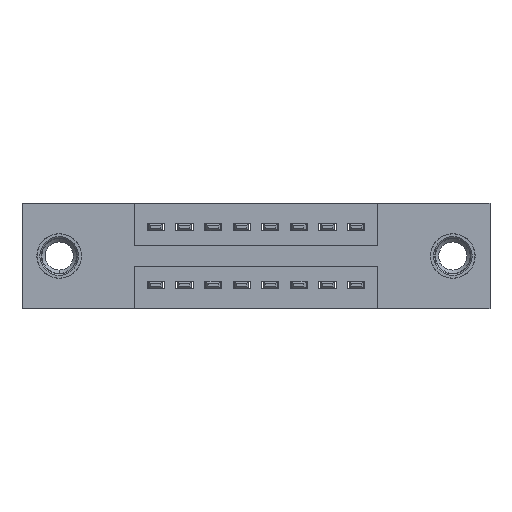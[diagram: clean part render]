
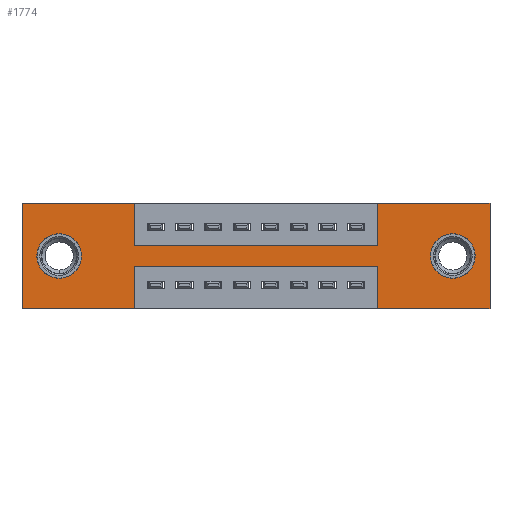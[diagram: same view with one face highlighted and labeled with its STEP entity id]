
A CAD part, front view. The second image highlights one B-rep face of the part: STEP entity #1774.
In plain terms, the highlighted planar face has unit normal (0, -1, 0).
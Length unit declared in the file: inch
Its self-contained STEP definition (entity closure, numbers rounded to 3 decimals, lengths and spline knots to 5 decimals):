
#6 = ORIENTED_EDGE ( 'NONE', *, *, #5524, .T. ) ;
#13 = VERTEX_POINT ( 'NONE', #3725 ) ;
#66 = EDGE_CURVE ( 'NONE', #8561, #3732, #9555, .T. ) ;
#76 = ORIENTED_EDGE ( 'NONE', *, *, #7674, .F. ) ;
#367 = ORIENTED_EDGE ( 'NONE', *, *, #10205, .F. ) ;
#395 = VERTEX_POINT ( 'NONE', #7832 ) ;
#459 = ORIENTED_EDGE ( 'NONE', *, *, #5177, .F. ) ;
#514 = LINE ( 'NONE', #8436, #5668 ) ;
#720 = DIRECTION ( 'NONE',  ( 1., 0., 0. ) ) ;
#758 = EDGE_CURVE ( 'NONE', #3732, #9157, #6215, .T. ) ;
#773 = FACE_BOUND ( 'NONE', #6918, .T. ) ;
#788 = ORIENTED_EDGE ( 'NONE', *, *, #1608, .T. ) ;
#1015 = VERTEX_POINT ( 'NONE', #11795 ) ;
#1145 = VECTOR ( 'NONE', #6794, 39.37008 ) ;
#1333 = CARTESIAN_POINT ( 'NONE',  ( 0., 0., 0. ) ) ;
#1350 = DIRECTION ( 'NONE',  ( 0., 1., 0. ) ) ;
#1471 = ORIENTED_EDGE ( 'NONE', *, *, #9600, .F. ) ;
#1476 = EDGE_CURVE ( 'NONE', #9157, #395, #10089, .T. ) ;
#1489 = DIRECTION ( 'NONE',  ( 0., 0., -1. ) ) ;
#1569 = VERTEX_POINT ( 'NONE', #2866 ) ;
#1586 = CARTESIAN_POINT ( 'NONE',  ( 1.2425, 0., 0. ) ) ;
#1608 = EDGE_CURVE ( 'NONE', #1569, #13, #11328, .T. ) ;
#1685 = CARTESIAN_POINT ( 'NONE',  ( 1.505, 0., -0.185 ) ) ;
#1750 = CIRCLE ( 'NONE', #9805, 0.078 ) ;
#1774 = ADVANCED_FACE ( 'NONE', ( #7945, #773, #5615 ), #3013, .T. ) ;
#1789 = CARTESIAN_POINT ( 'NONE',  ( 0., 0., 0. ) ) ;
#1961 = ORIENTED_EDGE ( 'NONE', *, *, #1476, .F. ) ;
#2021 = ORIENTED_EDGE ( 'NONE', *, *, #2684, .T. ) ;
#2031 = LINE ( 'NONE', #1333, #7217 ) ;
#2106 = ORIENTED_EDGE ( 'NONE', *, *, #9376, .F. ) ;
#2152 = EDGE_CURVE ( 'NONE', #13, #1569, #4315, .T. ) ;
#2191 = ORIENTED_EDGE ( 'NONE', *, *, #2152, .T. ) ;
#2216 = VERTEX_POINT ( 'NONE', #6932 ) ;
#2254 = CARTESIAN_POINT ( 'NONE',  ( 1.2425, 0., -0.22 ) ) ;
#2636 = ORIENTED_EDGE ( 'NONE', *, *, #10783, .F. ) ;
#2684 = EDGE_CURVE ( 'NONE', #5023, #7451, #8291, .T. ) ;
#2705 = LINE ( 'NONE', #7246, #4887 ) ;
#2793 = CARTESIAN_POINT ( 'NONE',  ( 1.2425, 0., -0.15 ) ) ;
#2866 = CARTESIAN_POINT ( 'NONE',  ( 1.505, 0., -0.263 ) ) ;
#2899 = DIRECTION ( 'NONE',  ( 0., 0., -1. ) ) ;
#2922 = VECTOR ( 'NONE', #720, 39.37008 ) ;
#2944 = AXIS2_PLACEMENT_3D ( 'NONE', #1685, #1350, #1489 ) ;
#3013 = PLANE ( 'NONE',  #8326 ) ;
#3107 = DIRECTION ( 'NONE',  ( 0., 0., -1. ) ) ;
#3128 = CARTESIAN_POINT ( 'NONE',  ( 0.13, 0., -0.185 ) ) ;
#3194 = DIRECTION ( 'NONE',  ( 0., 0., -1. ) ) ;
#3308 = DIRECTION ( 'NONE',  ( 0., -1., 0. ) ) ;
#3347 = CARTESIAN_POINT ( 'NONE',  ( 0., 0., -0.37 ) ) ;
#3351 = VERTEX_POINT ( 'NONE', #1586 ) ;
#3572 = VERTEX_POINT ( 'NONE', #11806 ) ;
#3608 = VECTOR ( 'NONE', #2899, 39.37008 ) ;
#3664 = CARTESIAN_POINT ( 'NONE',  ( 0.3925, 0., -0.37 ) ) ;
#3669 = VECTOR ( 'NONE', #4678, 39.37008 ) ;
#3725 = CARTESIAN_POINT ( 'NONE',  ( 1.505, 0., -0.107 ) ) ;
#3732 = VERTEX_POINT ( 'NONE', #2254 ) ;
#3815 = ORIENTED_EDGE ( 'NONE', *, *, #4090, .F. ) ;
#4055 = DIRECTION ( 'NONE',  ( 0., 0., 1. ) ) ;
#4090 = EDGE_CURVE ( 'NONE', #395, #11624, #11880, .T. ) ;
#4171 = ORIENTED_EDGE ( 'NONE', *, *, #66, .F. ) ;
#4315 = CIRCLE ( 'NONE', #8680, 0.078 ) ;
#4380 = CARTESIAN_POINT ( 'NONE',  ( 1.2425, 0., 0. ) ) ;
#4478 = CARTESIAN_POINT ( 'NONE',  ( 0., 0., -0.37 ) ) ;
#4615 = ORIENTED_EDGE ( 'NONE', *, *, #758, .F. ) ;
#4678 = DIRECTION ( 'NONE',  ( 0., 0., 1. ) ) ;
#4767 = EDGE_LOOP ( 'NONE', ( #2191, #788 ) ) ;
#4857 = CARTESIAN_POINT ( 'NONE',  ( 1.2425, 0., -0.37 ) ) ;
#4887 = VECTOR ( 'NONE', #11569, 39.37008 ) ;
#4925 = VECTOR ( 'NONE', #5820, 39.37008 ) ;
#5023 = VERTEX_POINT ( 'NONE', #11286 ) ;
#5134 = CARTESIAN_POINT ( 'NONE',  ( 0.3925, 0., -0.22 ) ) ;
#5177 = EDGE_CURVE ( 'NONE', #3351, #2216, #7677, .T. ) ;
#5264 = VERTEX_POINT ( 'NONE', #2793 ) ;
#5354 = AXIS2_PLACEMENT_3D ( 'NONE', #8125, #8090, #8054 ) ;
#5524 = EDGE_CURVE ( 'NONE', #7451, #5023, #1750, .T. ) ;
#5549 = CARTESIAN_POINT ( 'NONE',  ( 0.3925, 0., -0.15 ) ) ;
#5615 = FACE_OUTER_BOUND ( 'NONE', #7780, .T. ) ;
#5657 = LINE ( 'NONE', #5549, #2922 ) ;
#5668 = VECTOR ( 'NONE', #3107, 39.37008 ) ;
#5820 = DIRECTION ( 'NONE',  ( 0., 0., 1. ) ) ;
#5823 = LINE ( 'NONE', #1789, #3669 ) ;
#5928 = EDGE_CURVE ( 'NONE', #10672, #8561, #2705, .T. ) ;
#6215 = LINE ( 'NONE', #10726, #1145 ) ;
#6374 = CARTESIAN_POINT ( 'NONE',  ( 1.635, 0., 0. ) ) ;
#6794 = DIRECTION ( 'NONE',  ( -1., 0., 0. ) ) ;
#6808 = LINE ( 'NONE', #4380, #7065 ) ;
#6905 = EDGE_CURVE ( 'NONE', #1015, #10204, #2031, .T. ) ;
#6918 = EDGE_LOOP ( 'NONE', ( #2021, #6 ) ) ;
#6932 = CARTESIAN_POINT ( 'NONE',  ( 1.635, 0., 0. ) ) ;
#6963 = CARTESIAN_POINT ( 'NONE',  ( 1.635, 0., -0.37 ) ) ;
#7065 = VECTOR ( 'NONE', #8739, 39.37008 ) ;
#7217 = VECTOR ( 'NONE', #7816, 39.37008 ) ;
#7246 = CARTESIAN_POINT ( 'NONE',  ( 0., 0., -0.37 ) ) ;
#7286 = VECTOR ( 'NONE', #9884, 39.37008 ) ;
#7451 = VERTEX_POINT ( 'NONE', #8423 ) ;
#7674 = EDGE_CURVE ( 'NONE', #2216, #10672, #8265, .T. ) ;
#7677 = LINE ( 'NONE', #8065, #11735 ) ;
#7780 = EDGE_LOOP ( 'NONE', ( #1961, #4615, #4171, #10823, #76, #459, #2636, #367, #1471, #8094, #2106, #3815 ) ) ;
#7816 = DIRECTION ( 'NONE',  ( 1., 0., 0. ) ) ;
#7832 = CARTESIAN_POINT ( 'NONE',  ( 0.3925, 0., -0.37 ) ) ;
#7945 = FACE_BOUND ( 'NONE', #4767, .T. ) ;
#8054 = DIRECTION ( 'NONE',  ( 0., 0., 1. ) ) ;
#8065 = CARTESIAN_POINT ( 'NONE',  ( 0., 0., 0. ) ) ;
#8090 = DIRECTION ( 'NONE',  ( 0., 1., 0. ) ) ;
#8094 = ORIENTED_EDGE ( 'NONE', *, *, #6905, .F. ) ;
#8125 = CARTESIAN_POINT ( 'NONE',  ( 0.13, 0., -0.185 ) ) ;
#8265 = LINE ( 'NONE', #6374, #10593 ) ;
#8291 = CIRCLE ( 'NONE', #5354, 0.078 ) ;
#8326 = AXIS2_PLACEMENT_3D ( 'NONE', #3347, #3308, #3194 ) ;
#8423 = CARTESIAN_POINT ( 'NONE',  ( 0.13, 0., -0.263 ) ) ;
#8436 = CARTESIAN_POINT ( 'NONE',  ( 0.3925, 0., 0. ) ) ;
#8561 = VERTEX_POINT ( 'NONE', #10278 ) ;
#8680 = AXIS2_PLACEMENT_3D ( 'NONE', #9238, #9250, #9213 ) ;
#8739 = DIRECTION ( 'NONE',  ( 0., 0., 1. ) ) ;
#8992 = CARTESIAN_POINT ( 'NONE',  ( 0., 0., -0.37 ) ) ;
#9157 = VERTEX_POINT ( 'NONE', #5134 ) ;
#9213 = DIRECTION ( 'NONE',  ( 0., 0., -1. ) ) ;
#9238 = CARTESIAN_POINT ( 'NONE',  ( 1.505, 0., -0.185 ) ) ;
#9250 = DIRECTION ( 'NONE',  ( 0., 1., 0. ) ) ;
#9298 = DIRECTION ( 'NONE',  ( 0., 1., 0. ) ) ;
#9376 = EDGE_CURVE ( 'NONE', #11624, #1015, #5823, .T. ) ;
#9555 = LINE ( 'NONE', #4857, #4925 ) ;
#9600 = EDGE_CURVE ( 'NONE', #10204, #3572, #514, .T. ) ;
#9805 = AXIS2_PLACEMENT_3D ( 'NONE', #3128, #9298, #4055 ) ;
#9825 = DIRECTION ( 'NONE',  ( 0., 0., -1. ) ) ;
#9884 = DIRECTION ( 'NONE',  ( -1., 0., 0. ) ) ;
#10089 = LINE ( 'NONE', #3664, #3608 ) ;
#10204 = VERTEX_POINT ( 'NONE', #11628 ) ;
#10205 = EDGE_CURVE ( 'NONE', #3572, #5264, #5657, .T. ) ;
#10278 = CARTESIAN_POINT ( 'NONE',  ( 1.2425, 0., -0.37 ) ) ;
#10593 = VECTOR ( 'NONE', #9825, 39.37008 ) ;
#10672 = VERTEX_POINT ( 'NONE', #6963 ) ;
#10726 = CARTESIAN_POINT ( 'NONE',  ( 0.3925, 0., -0.22 ) ) ;
#10783 = EDGE_CURVE ( 'NONE', #5264, #3351, #6808, .T. ) ;
#10823 = ORIENTED_EDGE ( 'NONE', *, *, #5928, .F. ) ;
#11286 = CARTESIAN_POINT ( 'NONE',  ( 0.13, 0., -0.107 ) ) ;
#11328 = CIRCLE ( 'NONE', #2944, 0.078 ) ;
#11543 = DIRECTION ( 'NONE',  ( 1., 0., 0. ) ) ;
#11569 = DIRECTION ( 'NONE',  ( -1., 0., 0. ) ) ;
#11624 = VERTEX_POINT ( 'NONE', #4478 ) ;
#11628 = CARTESIAN_POINT ( 'NONE',  ( 0.3925, 0., 0. ) ) ;
#11735 = VECTOR ( 'NONE', #11543, 39.37008 ) ;
#11795 = CARTESIAN_POINT ( 'NONE',  ( 0., 0., 0. ) ) ;
#11806 = CARTESIAN_POINT ( 'NONE',  ( 0.3925, 0., -0.15 ) ) ;
#11880 = LINE ( 'NONE', #8992, #7286 ) ;
